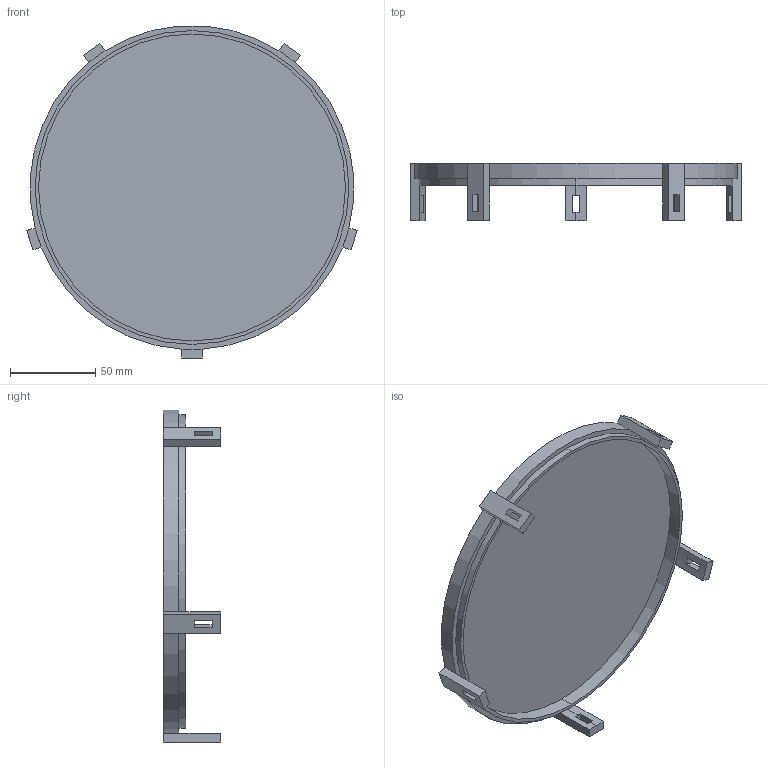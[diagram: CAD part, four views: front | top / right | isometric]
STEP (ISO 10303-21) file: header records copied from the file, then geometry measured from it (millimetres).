
FILE_DESCRIPTION (( 'STEP AP214' ), '1' );
FILE_NAME ('rear.STEP', '2013-12-19T18:59:35', ( '' ), ( '' ), 'SwSTEP 2.0', 'SolidWorks 2013', '' );
FILE_SCHEMA (( 'AUTOMOTIVE_DESIGN' ));
Length unit declared in the file: millimetre
Products named in the file (1): rear
Bounding box: 193.85 x 33.46 x 194.69 mm (x, y, z)
Volume: 166910.3 mm3; surface area: 74424.3 mm2
Topology: 1 solids, 1 shells, 59 faces, 158 edges, 102 vertices
Faces by surface type: plane 44, cylinder 15
Entity records: 1888 total; most frequent: DIRECTION 320, CARTESIAN_POINT 320, ORIENTED_EDGE 316, EDGE_CURVE 158, LINE 116, VECTOR 116, AXIS2_PLACEMENT_3D 102, VERTEX_POINT 102
